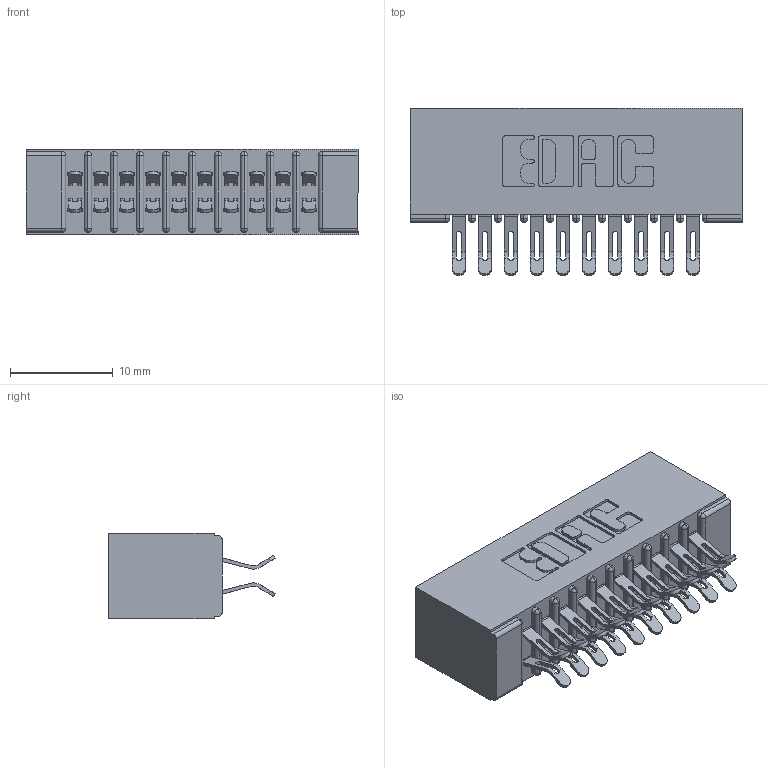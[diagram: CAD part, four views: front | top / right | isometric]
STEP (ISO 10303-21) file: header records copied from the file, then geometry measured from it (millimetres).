
FILE_DESCRIPTION (( 'STEP AP203' ), '1' );
FILE_NAME ('341-020-555-201.STEP', '2018-08-06T16:54:53', ( '' ), ( '' ), 'SwSTEP 2.0', 'SolidWorks 2016', '' );
FILE_SCHEMA (( 'CONFIG_CONTROL_DESIGN' ));
Length unit declared in the file: inch
Products named in the file (3): 341 Part_No Mounting Lugs; 341-292-001_341-292-155; 341-020-555-201
Assembly tree (21 placements, depth 2):
  341-020-555-201
    341 Part_No Mounting Lugs
    341-292-001_341-292-155  x20
Bounding box: 32.38 x 16.31 x 8.38 mm (x, y, z)
Volume: 2030.7 mm3; surface area: 4322.2 mm2
Topology: 21 solids, 21 shells, 1668 faces, 4962 edges, 3230 vertices
Faces by surface type: plane 904, cylinder 724, sphere 22, torus 18
Entity records: 16557 total; most frequent: CARTESIAN_POINT 2768, ORIENTED_EDGE 2736, DIRECTION 2698, EDGE_CURVE 1368, VECTOR 1058, LINE 1058, VERTEX_POINT 874, AXIS2_PLACEMENT_3D 820
